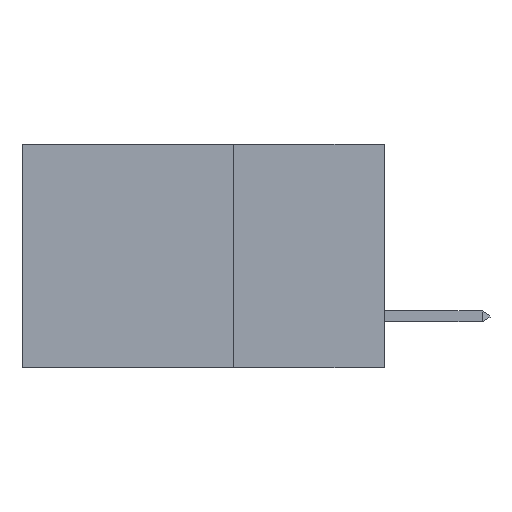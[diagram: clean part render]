
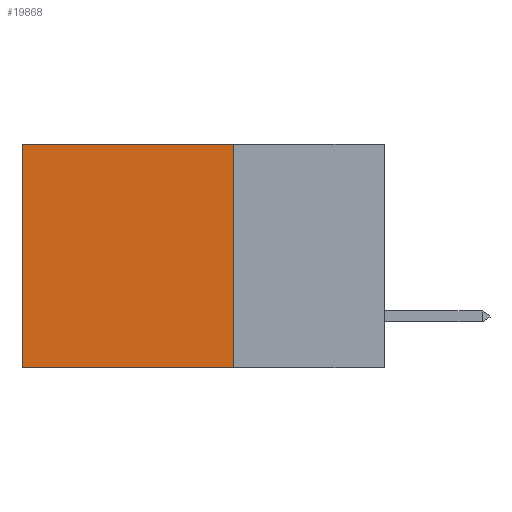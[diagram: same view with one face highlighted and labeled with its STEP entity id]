
A CAD part, left-side view. The second image highlights one B-rep face of the part: STEP entity #19868.
In plain terms, the highlighted planar face has unit normal (-1, 0, 0).
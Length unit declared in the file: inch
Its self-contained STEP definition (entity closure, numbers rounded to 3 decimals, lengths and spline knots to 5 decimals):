
#313 = ORIENTED_EDGE ( 'NONE', *, *, #13039, .T. ) ;
#549 = CARTESIAN_POINT ( 'NONE',  ( 0.2875, 0.25, 0. ) ) ;
#1704 = ORIENTED_EDGE ( 'NONE', *, *, #3434, .F. ) ;
#2570 = CARTESIAN_POINT ( 'NONE',  ( 0.2875, 0.25, 0. ) ) ;
#2900 = LINE ( 'NONE', #16249, #7716 ) ;
#3265 = VERTEX_POINT ( 'NONE', #17566 ) ;
#3434 = EDGE_CURVE ( 'NONE', #20289, #13875, #2900, .T. ) ;
#4204 = DIRECTION ( 'NONE',  ( 0., 1., 0. ) ) ;
#4611 = LINE ( 'NONE', #549, #8885 ) ;
#5218 = VECTOR ( 'NONE', #4204, 39.37008 ) ;
#6440 = PLANE ( 'NONE',  #11592 ) ;
#6914 = ORIENTED_EDGE ( 'NONE', *, *, #7774, .F. ) ;
#7370 = DIRECTION ( 'NONE',  ( 0., 0., -1. ) ) ;
#7404 = FACE_OUTER_BOUND ( 'NONE', #12970, .T. ) ;
#7450 = DIRECTION ( 'NONE',  ( 0., 0., -1. ) ) ;
#7716 = VECTOR ( 'NONE', #7370, 39.37008 ) ;
#7774 = EDGE_CURVE ( 'NONE', #13875, #8994, #9245, .T. ) ;
#8270 = DIRECTION ( 'NONE',  ( 0., 0., -1. ) ) ;
#8370 = VECTOR ( 'NONE', #7450, 39.37008 ) ;
#8885 = VECTOR ( 'NONE', #16716, 39.37008 ) ;
#8994 = VERTEX_POINT ( 'NONE', #11409 ) ;
#9245 = LINE ( 'NONE', #13160, #5218 ) ;
#11107 = EDGE_CURVE ( 'NONE', #3265, #8994, #13107, .T. ) ;
#11409 = CARTESIAN_POINT ( 'NONE',  ( 0.2875, 0.6, -0.37 ) ) ;
#11592 = AXIS2_PLACEMENT_3D ( 'NONE', #2570, #18869, #8270 ) ;
#12397 = ORIENTED_EDGE ( 'NONE', *, *, #11107, .T. ) ;
#12789 = CARTESIAN_POINT ( 'NONE',  ( 0.2875, 0.6, 0. ) ) ;
#12970 = EDGE_LOOP ( 'NONE', ( #12397, #6914, #1704, #313 ) ) ;
#13039 = EDGE_CURVE ( 'NONE', #20289, #3265, #4611, .T. ) ;
#13107 = LINE ( 'NONE', #12789, #8370 ) ;
#13160 = CARTESIAN_POINT ( 'NONE',  ( 0.2875, 0.25, -0.37 ) ) ;
#13875 = VERTEX_POINT ( 'NONE', #21749 ) ;
#16249 = CARTESIAN_POINT ( 'NONE',  ( 0.2875, 0.25, 0. ) ) ;
#16716 = DIRECTION ( 'NONE',  ( 0., 1., 0. ) ) ;
#17566 = CARTESIAN_POINT ( 'NONE',  ( 0.2875, 0.6, 0. ) ) ;
#18869 = DIRECTION ( 'NONE',  ( 1., 0., 0. ) ) ;
#19868 = ADVANCED_FACE ( 'NONE', ( #7404 ), #6440, .F. ) ;
#20083 = CARTESIAN_POINT ( 'NONE',  ( 0.2875, 0.25, 0. ) ) ;
#20289 = VERTEX_POINT ( 'NONE', #20083 ) ;
#21749 = CARTESIAN_POINT ( 'NONE',  ( 0.2875, 0.25, -0.37 ) ) ;
